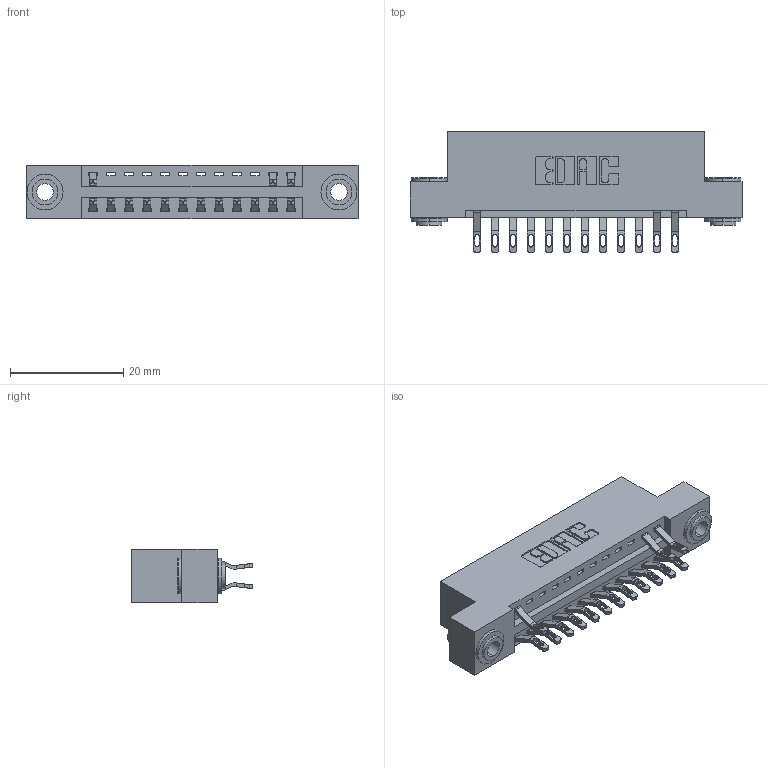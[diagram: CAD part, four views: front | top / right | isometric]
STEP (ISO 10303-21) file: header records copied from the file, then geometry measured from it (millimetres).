
FILE_DESCRIPTION (( 'STEP AP203' ), '1' );
FILE_NAME ('346-024-555-203.STEP', '2018-08-21T04:06:10', ( '' ), ( '' ), 'SwSTEP 2.0', 'SolidWorks 2016', '' );
FILE_SCHEMA (( 'CONFIG_CONTROL_DESIGN' ));
Length unit declared in the file: inch
Products named in the file (4): 346 Part_Flush Mounting Lugs - 0.156 Dia-TH; 345-292-001_555 Tail; 345-250-002_345-250-002-102; 346-024-555-203
Assembly tree (18 placements, depth 2):
  346-024-555-203
    346 Part_Flush Mounting Lugs - 0.156 Dia-TH
    345-292-001_555 Tail  x15
    345-250-002_345-250-002-102  x2
Bounding box: 58.67 x 21.46 x 9.4 mm (x, y, z)
Volume: 5470.4 mm3; surface area: 6950 mm2
Topology: 18 solids, 18 shells, 1084 faces, 3339 edges, 2222 vertices
Faces by surface type: plane 626, cylinder 450, cone 8
Entity records: 12558 total; most frequent: CARTESIAN_POINT 2160, ORIENTED_EDGE 2066, DIRECTION 1945, EDGE_CURVE 1033, VECTOR 809, LINE 809, VERTEX_POINT 686, AXIS2_PLACEMENT_3D 568
